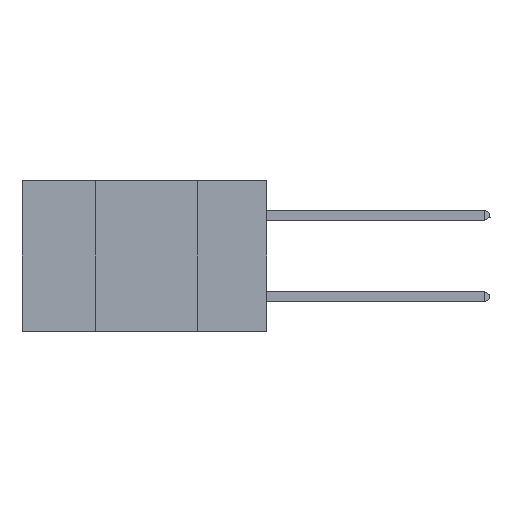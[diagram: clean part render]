
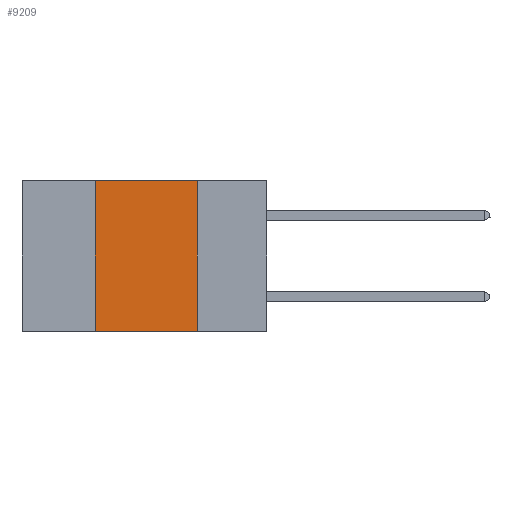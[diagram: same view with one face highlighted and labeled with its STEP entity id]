
A CAD part, left-side view. The second image highlights one B-rep face of the part: STEP entity #9209.
In plain terms, the highlighted planar face has unit normal (-1, 0, 0).
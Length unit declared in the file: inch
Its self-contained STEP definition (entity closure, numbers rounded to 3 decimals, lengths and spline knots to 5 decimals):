
#451 = LINE ( 'NONE', #10211, #15142 ) ;
#2315 = ORIENTED_EDGE ( 'NONE', *, *, #20281, .F. ) ;
#2699 = CARTESIAN_POINT ( 'NONE',  ( 0., 0.17, 0. ) ) ;
#4396 = DIRECTION ( 'NONE',  ( 0., -1., 0. ) ) ;
#5027 = DIRECTION ( 'NONE',  ( 1., 0., 0. ) ) ;
#5038 = CARTESIAN_POINT ( 'NONE',  ( 0., 0.42, 0. ) ) ;
#6122 = EDGE_CURVE ( 'NONE', #25216, #24585, #13933, .T. ) ;
#6313 = CARTESIAN_POINT ( 'NONE',  ( 0., 0.17, -0.37 ) ) ;
#6726 = DIRECTION ( 'NONE',  ( 0., 0., 1. ) ) ;
#7806 = VERTEX_POINT ( 'NONE', #6313 ) ;
#8772 = ORIENTED_EDGE ( 'NONE', *, *, #25000, .T. ) ;
#9098 = CARTESIAN_POINT ( 'NONE',  ( 0., 0.42, -0.37 ) ) ;
#9209 = ADVANCED_FACE ( 'NONE', ( #21432 ), #10746, .F. ) ;
#9252 = AXIS2_PLACEMENT_3D ( 'NONE', #12790, #5027, #16539 ) ;
#9378 = VECTOR ( 'NONE', #6726, 39.37008 ) ;
#10211 = CARTESIAN_POINT ( 'NONE',  ( 0., 0.6, -0.37 ) ) ;
#10746 = PLANE ( 'NONE',  #9252 ) ;
#11181 = VECTOR ( 'NONE', #24140, 39.37008 ) ;
#11835 = CARTESIAN_POINT ( 'NONE',  ( 0., 0.6, 0. ) ) ;
#12320 = LINE ( 'NONE', #11835, #17504 ) ;
#12790 = CARTESIAN_POINT ( 'NONE',  ( 0., 0.6, 0. ) ) ;
#13623 = ORIENTED_EDGE ( 'NONE', *, *, #16430, .F. ) ;
#13777 = DIRECTION ( 'NONE',  ( 0., -1., 0. ) ) ;
#13933 = LINE ( 'NONE', #14475, #9378 ) ;
#14475 = CARTESIAN_POINT ( 'NONE',  ( 0., 0.42, 0. ) ) ;
#15142 = VECTOR ( 'NONE', #4396, 39.37008 ) ;
#16430 = EDGE_CURVE ( 'NONE', #22498, #7806, #17569, .T. ) ;
#16504 = ORIENTED_EDGE ( 'NONE', *, *, #6122, .F. ) ;
#16539 = DIRECTION ( 'NONE',  ( 0., 0., -1. ) ) ;
#17504 = VECTOR ( 'NONE', #13777, 39.37008 ) ;
#17569 = LINE ( 'NONE', #22352, #11181 ) ;
#19086 = EDGE_LOOP ( 'NONE', ( #13623, #2315, #16504, #8772 ) ) ;
#20281 = EDGE_CURVE ( 'NONE', #24585, #22498, #12320, .T. ) ;
#21432 = FACE_OUTER_BOUND ( 'NONE', #19086, .T. ) ;
#22352 = CARTESIAN_POINT ( 'NONE',  ( 0., 0.17, 0. ) ) ;
#22498 = VERTEX_POINT ( 'NONE', #2699 ) ;
#24140 = DIRECTION ( 'NONE',  ( 0., 0., -1. ) ) ;
#24585 = VERTEX_POINT ( 'NONE', #5038 ) ;
#25000 = EDGE_CURVE ( 'NONE', #25216, #7806, #451, .T. ) ;
#25216 = VERTEX_POINT ( 'NONE', #9098 ) ;
